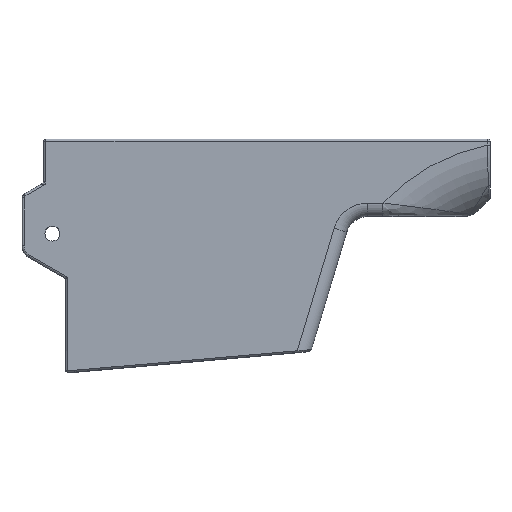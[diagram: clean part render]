
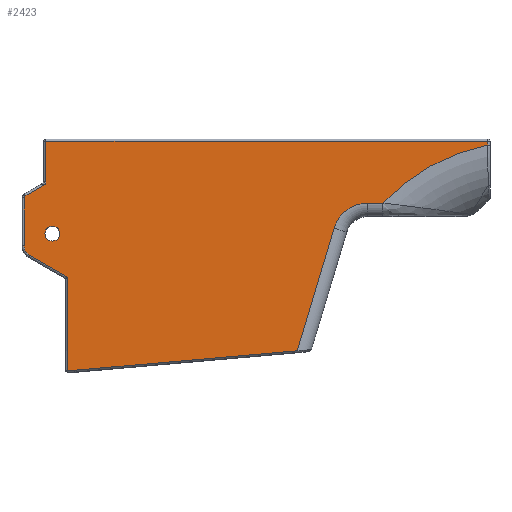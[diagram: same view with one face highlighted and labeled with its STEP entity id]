
A CAD part, top view. The second image highlights one B-rep face of the part: STEP entity #2423.
In plain terms, the highlighted planar face has unit normal (0, 0, 1).
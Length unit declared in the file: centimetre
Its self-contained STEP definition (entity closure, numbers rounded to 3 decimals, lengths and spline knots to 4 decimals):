
#51=CIRCLE($,#2585,4.5);
#52=CIRCLE($,#2587,0.051);
#53=CIRCLE($,#2588,0.251);
#54=CIRCLE($,#2589,0.8);
#55=CIRCLE($,#2590,0.17);
#195=FACE_BOUND($,#446,.T.);
#217=PLANE($,#2586);
#290=FACE_OUTER_BOUND($,#445,.T.);
#445=EDGE_LOOP($,(#1808,#1809,#1810,#1811,#1812,#1813,#1814,#1815,#1816,
#1817,#1818,#1819,#1820,#1821,#1822));
#446=EDGE_LOOP($,(#1823));
#617=LINE($,#4006,#795);
#633=LINE($,#4184,#811);
#634=LINE($,#4186,#812);
#635=LINE($,#4188,#813);
#636=LINE($,#4192,#814);
#637=LINE($,#4196,#815);
#638=LINE($,#4198,#816);
#639=LINE($,#4200,#817);
#640=LINE($,#4207,#818);
#641=LINE($,#4210,#819);
#795=VECTOR($,#2862,0.0873);
#811=VECTOR($,#2918,10.0578);
#812=VECTOR($,#2919,0.9736);
#813=VECTOR($,#2920,0.5502);
#814=VECTOR($,#2923,1.0887);
#815=VECTOR($,#2926,1.0027);
#816=VECTOR($,#2927,2.1311);
#817=VECTOR($,#2928,5.226);
#818=VECTOR($,#2929,2.9126);
#819=VECTOR($,#2932,0.3447);
#972=B_SPLINE_CURVE_WITH_KNOTS($,3,(#4202,#4203,#4204,#4205),
 .UNSPECIFIED.,.F.,.F.,(4,4),(1.5215,1.5708),
 .UNSPECIFIED.);
#1075=VERTEX_POINT($,#3996);
#1077=VERTEX_POINT($,#4004);
#1103=VERTEX_POINT($,#4168);
#1105=VERTEX_POINT($,#4183);
#1106=VERTEX_POINT($,#4185);
#1107=VERTEX_POINT($,#4187);
#1108=VERTEX_POINT($,#4189);
#1109=VERTEX_POINT($,#4191);
#1110=VERTEX_POINT($,#4193);
#1111=VERTEX_POINT($,#4195);
#1112=VERTEX_POINT($,#4197);
#1113=VERTEX_POINT($,#4199);
#1114=VERTEX_POINT($,#4201);
#1115=VERTEX_POINT($,#4206);
#1116=VERTEX_POINT($,#4208);
#1117=VERTEX_POINT($,#4211);
#1327=EDGE_CURVE($,#1077,#1075,#617,.T.);
#1363=EDGE_CURVE($,#1075,#1103,#51,.T.);
#1366=EDGE_CURVE($,#1105,#1077,#633,.T.);
#1367=EDGE_CURVE($,#1106,#1105,#634,.T.);
#1368=EDGE_CURVE($,#1107,#1106,#635,.T.);
#1369=EDGE_CURVE($,#1108,#1107,#52,.T.);
#1370=EDGE_CURVE($,#1109,#1108,#636,.T.);
#1371=EDGE_CURVE($,#1110,#1109,#53,.T.);
#1372=EDGE_CURVE($,#1111,#1110,#637,.T.);
#1373=EDGE_CURVE($,#1112,#1111,#638,.T.);
#1374=EDGE_CURVE($,#1113,#1112,#639,.T.);
#1375=EDGE_CURVE($,#1114,#1113,#972,.T.);
#1376=EDGE_CURVE($,#1115,#1114,#640,.T.);
#1377=EDGE_CURVE($,#1116,#1115,#54,.T.);
#1378=EDGE_CURVE($,#1103,#1116,#641,.T.);
#1379=EDGE_CURVE($,#1117,#1117,#55,.F.);
#1808=ORIENTED_EDGE($,*,*,#1327,.F.);
#1809=ORIENTED_EDGE($,*,*,#1366,.F.);
#1810=ORIENTED_EDGE($,*,*,#1367,.F.);
#1811=ORIENTED_EDGE($,*,*,#1368,.F.);
#1812=ORIENTED_EDGE($,*,*,#1369,.F.);
#1813=ORIENTED_EDGE($,*,*,#1370,.F.);
#1814=ORIENTED_EDGE($,*,*,#1371,.F.);
#1815=ORIENTED_EDGE($,*,*,#1372,.F.);
#1816=ORIENTED_EDGE($,*,*,#1373,.F.);
#1817=ORIENTED_EDGE($,*,*,#1374,.F.);
#1818=ORIENTED_EDGE($,*,*,#1375,.F.);
#1819=ORIENTED_EDGE($,*,*,#1376,.F.);
#1820=ORIENTED_EDGE($,*,*,#1377,.F.);
#1821=ORIENTED_EDGE($,*,*,#1378,.F.);
#1822=ORIENTED_EDGE($,*,*,#1363,.F.);
#1823=ORIENTED_EDGE($,*,*,#1379,.T.);
#2423=ADVANCED_FACE($,(#290,#195),#217,.F.);
#2585=AXIS2_PLACEMENT_3D($,#4169,#2914,#2915);
#2586=AXIS2_PLACEMENT_3D($,#4182,#2916,#2917);
#2587=AXIS2_PLACEMENT_3D($,#4190,#2921,#2922);
#2588=AXIS2_PLACEMENT_3D($,#4194,#2924,#2925);
#2589=AXIS2_PLACEMENT_3D($,#4209,#2930,#2931);
#2590=AXIS2_PLACEMENT_3D($,#4212,#2933,#2934);
#2862=DIRECTION($,(0.,-1.,0.));
#2914=DIRECTION('center_axis',(0.,0.,
1.));
#2915=DIRECTION('ref_axis',(-0.811,0.585,0.));
#2916=DIRECTION('center_axis',(0.,0.,
-1.));
#2917=DIRECTION('ref_axis',(0.,1.,0.));
#2918=DIRECTION($,(1.,0.,0.));
#2919=DIRECTION($,(0.,1.,0.));
#2920=DIRECTION($,(0.866,0.5,0.));
#2921=DIRECTION('center_axis',(0.,0.,
-1.));
#2922=DIRECTION('ref_axis',(-1.,0.,0.));
#2923=DIRECTION($,(0.,1.,0.));
#2924=DIRECTION('center_axis',(0.,0.,
-1.));
#2925=DIRECTION('ref_axis',(-0.866,-0.5,0.));
#2926=DIRECTION($,(-0.866,0.5,0.));
#2927=DIRECTION($,(0.,1.,0.));
#2928=DIRECTION($,(-0.996,-0.087,0.));
#2929=DIRECTION($,(-0.287,-0.958,0.));
#2930=DIRECTION('center_axis',(0.,0.,
1.));
#2931=DIRECTION('ref_axis',(-0.597,0.802,0.));
#2932=DIRECTION($,(-1.,0.,0.));
#2933=DIRECTION('center_axis',(0.,0.,
1.));
#2934=DIRECTION('ref_axis',(1.,0.,0.));
#3996=CARTESIAN_POINT('',(1.1178,-0.9663,-28.));
#4004=CARTESIAN_POINT('',(1.1178,-0.879,-28.));
#4006=CARTESIAN_POINT($,(1.1178,-3.3205,-28.));
#4168=CARTESIAN_POINT('',(-1.2702,-2.2877,-28.));
#4169=CARTESIAN_POINT('Origin',(2.,-5.379,-28.));
#4182=CARTESIAN_POINT('Origin',(-4.47,-3.454,-28.));
#4183=CARTESIAN_POINT('',(-8.94,-0.879,-28.));
#4184=CARTESIAN_POINT($,(-4.4407,-0.879,-28.));
#4185=CARTESIAN_POINT('',(-8.94,-1.8526,-28.));
#4186=CARTESIAN_POINT($,(-8.94,-1.6415,-28.));
#4187=CARTESIAN_POINT('',(-9.4165,-2.1277,-28.));
#4188=CARTESIAN_POINT($,(-7.8087,-1.1994,-28.));
#4189=CARTESIAN_POINT('',(-9.4338,-2.166,-28.));
#4190=CARTESIAN_POINT('Origin',(-9.3828,-2.166,-28.));
#4191=CARTESIAN_POINT('',(-9.4338,-3.2547,-28.));
#4192=CARTESIAN_POINT($,(-9.4338,-3.0677,-28.));
#4193=CARTESIAN_POINT('',(-9.3083,-3.472,-28.));
#4194=CARTESIAN_POINT('Origin',(-9.1828,-3.2547,-28.));
#4195=CARTESIAN_POINT('',(-8.44,-3.9734,-28.));
#4196=CARTESIAN_POINT($,(-7.5497,-4.4874,-28.));
#4197=CARTESIAN_POINT('',(-8.44,-6.1044,-28.));
#4198=CARTESIAN_POINT($,(-8.44,-3.8892,-28.));
#4199=CARTESIAN_POINT('',(-3.2339,-5.649,-28.));
#4200=CARTESIAN_POINT($,(-4.001,-5.7161,-28.));
#4201=CARTESIAN_POINT('',(-3.2181,-5.6476,-28.));
#4202=CARTESIAN_POINT('Ctrl Pts',(-3.2181,-5.6476,-28.));
#4203=CARTESIAN_POINT('Ctrl Pts',(-3.2234,-5.648,-28.));
#4204=CARTESIAN_POINT('Ctrl Pts',(-3.2287,-5.6485,-28.));
#4205=CARTESIAN_POINT('Ctrl Pts',(-3.2339,-5.649,-28.));
#4206=CARTESIAN_POINT('',(-2.3811,-2.8578,-28.));
#4207=CARTESIAN_POINT($,(-2.5836,-3.5327,-28.));
#4208=CARTESIAN_POINT('',(-1.6149,-2.2877,-28.));
#4209=CARTESIAN_POINT('Origin',(-1.6149,-3.0877,-28.));
#4210=CARTESIAN_POINT($,(-1.9118,-2.2877,-28.));
#4211=CARTESIAN_POINT('',(-8.96,-2.9815,-28.));
#4212=CARTESIAN_POINT('Origin',(-8.79,-2.9815,-28.));
